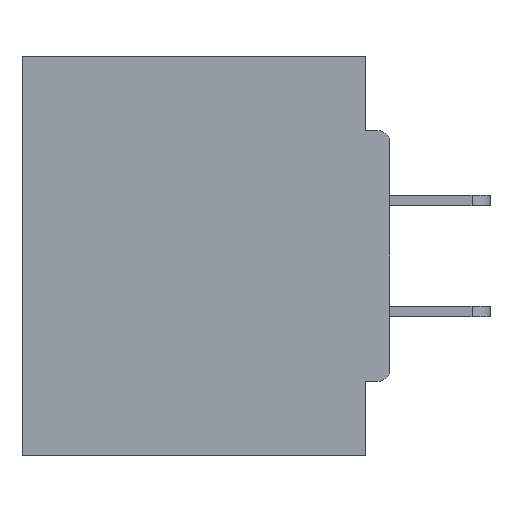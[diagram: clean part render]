
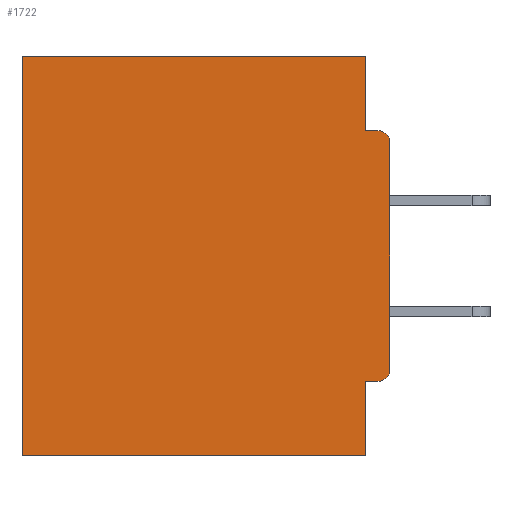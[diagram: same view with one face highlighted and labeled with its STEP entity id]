
A CAD part, left-side view. The second image highlights one B-rep face of the part: STEP entity #1722.
In plain terms, the highlighted planar face has unit normal (-1, 0, 0).
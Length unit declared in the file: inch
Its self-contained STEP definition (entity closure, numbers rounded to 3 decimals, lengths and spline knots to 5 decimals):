
#1278 = EDGE_CURVE ( 'NONE', #28557, #30584, #3220, .T. ) ;
#1722 = ADVANCED_FACE ( 'NONE', ( #14060 ), #21254, .F. ) ;
#1728 = CARTESIAN_POINT ( 'NONE',  ( 0.298, 0.031, 0. ) ) ;
#1780 = ORIENTED_EDGE ( 'NONE', *, *, #29778, .T. ) ;
#2029 = CIRCLE ( 'NONE', #4210, 0.015 ) ;
#3220 = LINE ( 'NONE', #27511, #24658 ) ;
#3592 = AXIS2_PLACEMENT_3D ( 'NONE', #16016, #15903, #26421 ) ;
#4210 = AXIS2_PLACEMENT_3D ( 'NONE', #23845, #24077, #23965 ) ;
#4260 = VECTOR ( 'NONE', #26642, 39.37008 ) ;
#4598 = CARTESIAN_POINT ( 'NONE',  ( 0.298, 0., 0. ) ) ;
#4903 = CARTESIAN_POINT ( 'NONE',  ( 0.298, 0.031, -0.4065 ) ) ;
#5232 = LINE ( 'NONE', #4598, #16593 ) ;
#5286 = ORIENTED_EDGE ( 'NONE', *, *, #1278, .T. ) ;
#5310 = VERTEX_POINT ( 'NONE', #29793 ) ;
#5372 = VERTEX_POINT ( 'NONE', #22830 ) ;
#5759 = DIRECTION ( 'NONE',  ( 0., 0., -1. ) ) ;
#5959 = EDGE_CURVE ( 'NONE', #5310, #30584, #21665, .T. ) ;
#6296 = LINE ( 'NONE', #14312, #22881 ) ;
#6715 = ORIENTED_EDGE ( 'NONE', *, *, #25077, .F. ) ;
#7476 = DIRECTION ( 'NONE',  ( 0., 1., 0. ) ) ;
#7899 = DIRECTION ( 'NONE',  ( 0., 1., 0. ) ) ;
#8303 = LINE ( 'NONE', #13615, #4260 ) ;
#8792 = CARTESIAN_POINT ( 'NONE',  ( 0.298, 0., -0.1085 ) ) ;
#9194 = EDGE_LOOP ( 'NONE', ( #10475, #30522, #6715, #16248, #5286, #18848, #10844, #20100, #1780, #14971 ) ) ;
#9825 = EDGE_CURVE ( 'NONE', #21088, #16972, #5232, .T. ) ;
#10475 = ORIENTED_EDGE ( 'NONE', *, *, #30194, .T. ) ;
#10844 = ORIENTED_EDGE ( 'NONE', *, *, #26464, .F. ) ;
#11131 = VECTOR ( 'NONE', #7899, 39.37008 ) ;
#12271 = DIRECTION ( 'NONE',  ( 0., 1., 0. ) ) ;
#12584 = DIRECTION ( 'NONE',  ( 0., 0., -1. ) ) ;
#13094 = CARTESIAN_POINT ( 'NONE',  ( 0.298, 0.46, -0.5 ) ) ;
#13180 = VERTEX_POINT ( 'NONE', #22267 ) ;
#13615 = CARTESIAN_POINT ( 'NONE',  ( 0.298, 0.031, -0.5 ) ) ;
#13668 = CARTESIAN_POINT ( 'NONE',  ( 0.298, 0., 0. ) ) ;
#14060 = FACE_OUTER_BOUND ( 'NONE', #9194, .T. ) ;
#14312 = CARTESIAN_POINT ( 'NONE',  ( 0.298, 0., -0.0935 ) ) ;
#14971 = ORIENTED_EDGE ( 'NONE', *, *, #9825, .F. ) ;
#14991 = DIRECTION ( 'NONE',  ( 0., -1., 0. ) ) ;
#15903 = DIRECTION ( 'NONE',  ( -1., 0., 0. ) ) ;
#16016 = CARTESIAN_POINT ( 'NONE',  ( 0.298, 0.015, -0.1085 ) ) ;
#16056 = DIRECTION ( 'NONE',  ( 1., 0., 0. ) ) ;
#16248 = ORIENTED_EDGE ( 'NONE', *, *, #24763, .T. ) ;
#16593 = VECTOR ( 'NONE', #12584, 39.37008 ) ;
#16972 = VERTEX_POINT ( 'NONE', #27192 ) ;
#18848 = ORIENTED_EDGE ( 'NONE', *, *, #5959, .F. ) ;
#20014 = CARTESIAN_POINT ( 'NONE',  ( 0.298, 0., -0.5 ) ) ;
#20100 = ORIENTED_EDGE ( 'NONE', *, *, #26569, .F. ) ;
#20365 = CARTESIAN_POINT ( 'NONE',  ( 0.298, 0., -0.4065 ) ) ;
#20487 = AXIS2_PLACEMENT_3D ( 'NONE', #13668, #16056, #5759 ) ;
#20738 = CARTESIAN_POINT ( 'NONE',  ( 0.298, 0.46, 0. ) ) ;
#20951 = LINE ( 'NONE', #22991, #32348 ) ;
#21088 = VERTEX_POINT ( 'NONE', #8792 ) ;
#21254 = PLANE ( 'NONE',  #20487 ) ;
#21292 = DIRECTION ( 'NONE',  ( 0., 0., -1. ) ) ;
#21665 = LINE ( 'NONE', #20014, #33443 ) ;
#22267 = CARTESIAN_POINT ( 'NONE',  ( 0.298, 0.031, -0.0935 ) ) ;
#22830 = CARTESIAN_POINT ( 'NONE',  ( 0.298, 0.015, -0.4065 ) ) ;
#22881 = VECTOR ( 'NONE', #14991, 39.37008 ) ;
#22991 = CARTESIAN_POINT ( 'NONE',  ( 0.298, 0., 0. ) ) ;
#23740 = LINE ( 'NONE', #23772, #26178 ) ;
#23772 = CARTESIAN_POINT ( 'NONE',  ( 0.298, 0.031, -0.5 ) ) ;
#23845 = CARTESIAN_POINT ( 'NONE',  ( 0.298, 0.015, -0.3915 ) ) ;
#23965 = DIRECTION ( 'NONE',  ( 0., 0., -1. ) ) ;
#24077 = DIRECTION ( 'NONE',  ( -1., 0., 0. ) ) ;
#24466 = VERTEX_POINT ( 'NONE', #26432 ) ;
#24658 = VECTOR ( 'NONE', #30022, 39.37008 ) ;
#24763 = EDGE_CURVE ( 'NONE', #30558, #28557, #20951, .T. ) ;
#25077 = EDGE_CURVE ( 'NONE', #30558, #13180, #23740, .T. ) ;
#26178 = VECTOR ( 'NONE', #21292, 39.37008 ) ;
#26421 = DIRECTION ( 'NONE',  ( 0., 0., -1. ) ) ;
#26432 = CARTESIAN_POINT ( 'NONE',  ( 0.298, 0.015, -0.0935 ) ) ;
#26464 = EDGE_CURVE ( 'NONE', #28152, #5310, #8303, .T. ) ;
#26569 = EDGE_CURVE ( 'NONE', #5372, #28152, #31861, .T. ) ;
#26642 = DIRECTION ( 'NONE',  ( 0., 0., -1. ) ) ;
#27192 = CARTESIAN_POINT ( 'NONE',  ( 0.298, 0., -0.3915 ) ) ;
#27511 = CARTESIAN_POINT ( 'NONE',  ( 0.298, 0.46, 0. ) ) ;
#28152 = VERTEX_POINT ( 'NONE', #4903 ) ;
#28557 = VERTEX_POINT ( 'NONE', #20738 ) ;
#29778 = EDGE_CURVE ( 'NONE', #5372, #16972, #2029, .T. ) ;
#29793 = CARTESIAN_POINT ( 'NONE',  ( 0.298, 0.031, -0.5 ) ) ;
#29958 = CIRCLE ( 'NONE', #3592, 0.015 ) ;
#30022 = DIRECTION ( 'NONE',  ( 0., 0., -1. ) ) ;
#30194 = EDGE_CURVE ( 'NONE', #21088, #24466, #29958, .T. ) ;
#30522 = ORIENTED_EDGE ( 'NONE', *, *, #33263, .F. ) ;
#30558 = VERTEX_POINT ( 'NONE', #1728 ) ;
#30584 = VERTEX_POINT ( 'NONE', #13094 ) ;
#31861 = LINE ( 'NONE', #20365, #11131 ) ;
#32348 = VECTOR ( 'NONE', #7476, 39.37008 ) ;
#33263 = EDGE_CURVE ( 'NONE', #13180, #24466, #6296, .T. ) ;
#33443 = VECTOR ( 'NONE', #12271, 39.37008 ) ;
